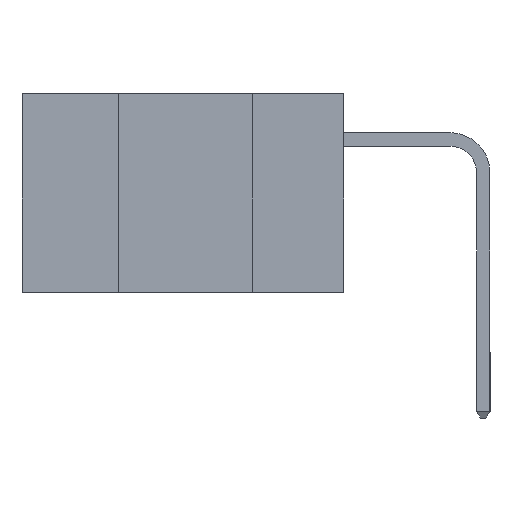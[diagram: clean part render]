
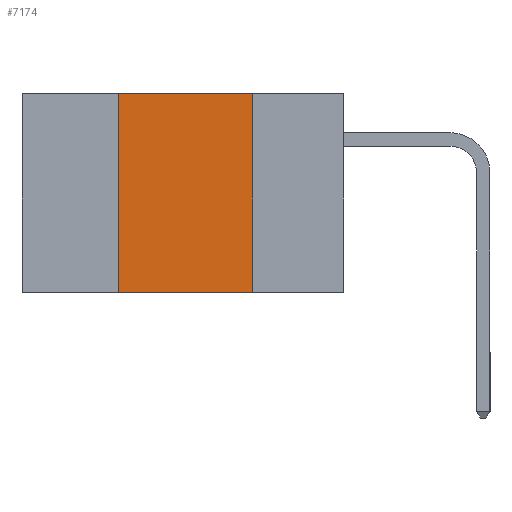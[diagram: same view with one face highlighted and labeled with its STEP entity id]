
A CAD part, left-side view. The second image highlights one B-rep face of the part: STEP entity #7174.
In plain terms, the highlighted planar face has unit normal (-1, 0, 0).
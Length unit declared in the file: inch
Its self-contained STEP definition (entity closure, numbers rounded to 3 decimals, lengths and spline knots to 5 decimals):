
#271 = DIRECTION ( 'NONE',  ( 0., -1., 0. ) ) ;
#311 = VERTEX_POINT ( 'NONE', #6300 ) ;
#550 = AXIS2_PLACEMENT_3D ( 'NONE', #8020, #4889, #9214 ) ;
#1442 = VECTOR ( 'NONE', #2116, 39.37008 ) ;
#1546 = ORIENTED_EDGE ( 'NONE', *, *, #4693, .T. ) ;
#2116 = DIRECTION ( 'NONE',  ( 0., 0., -1. ) ) ;
#2227 = DIRECTION ( 'NONE',  ( 0., 0., 1. ) ) ;
#2365 = CARTESIAN_POINT ( 'NONE',  ( 0., 0.42, -0.37 ) ) ;
#2449 = LINE ( 'NONE', #5404, #10309 ) ;
#3277 = EDGE_CURVE ( 'NONE', #311, #11477, #10362, .T. ) ;
#4693 = EDGE_CURVE ( 'NONE', #11360, #8022, #2449, .T. ) ;
#4889 = DIRECTION ( 'NONE',  ( 1., 0., 0. ) ) ;
#5208 = DIRECTION ( 'NONE',  ( 0., -1., 0. ) ) ;
#5230 = CARTESIAN_POINT ( 'NONE',  ( 0., 0.17, -0.37 ) ) ;
#5346 = EDGE_LOOP ( 'NONE', ( #12552, #11340, #6951, #1546 ) ) ;
#5404 = CARTESIAN_POINT ( 'NONE',  ( 0., 0.6, -0.37 ) ) ;
#5969 = PLANE ( 'NONE',  #550 ) ;
#6300 = CARTESIAN_POINT ( 'NONE',  ( 0., 0.42, 0. ) ) ;
#6310 = CARTESIAN_POINT ( 'NONE',  ( 0., 0.42, -0.37 ) ) ;
#6951 = ORIENTED_EDGE ( 'NONE', *, *, #7745, .F. ) ;
#7174 = ADVANCED_FACE ( 'NONE', ( #12876 ), #5969, .F. ) ;
#7241 = VECTOR ( 'NONE', #2227, 39.37008 ) ;
#7745 = EDGE_CURVE ( 'NONE', #11360, #311, #11630, .T. ) ;
#8020 = CARTESIAN_POINT ( 'NONE',  ( 0., 0.6, 0. ) ) ;
#8022 = VERTEX_POINT ( 'NONE', #5230 ) ;
#8134 = LINE ( 'NONE', #10101, #1442 ) ;
#8753 = EDGE_CURVE ( 'NONE', #11477, #8022, #8134, .T. ) ;
#9072 = VECTOR ( 'NONE', #5208, 39.37008 ) ;
#9214 = DIRECTION ( 'NONE',  ( 0., 0., -1. ) ) ;
#9627 = CARTESIAN_POINT ( 'NONE',  ( 0., 0.17, 0. ) ) ;
#10101 = CARTESIAN_POINT ( 'NONE',  ( 0., 0.17, -0.37 ) ) ;
#10309 = VECTOR ( 'NONE', #271, 39.37008 ) ;
#10362 = LINE ( 'NONE', #10427, #9072 ) ;
#10427 = CARTESIAN_POINT ( 'NONE',  ( 0., 0.6, 0. ) ) ;
#11340 = ORIENTED_EDGE ( 'NONE', *, *, #3277, .F. ) ;
#11360 = VERTEX_POINT ( 'NONE', #6310 ) ;
#11477 = VERTEX_POINT ( 'NONE', #9627 ) ;
#11630 = LINE ( 'NONE', #2365, #7241 ) ;
#12552 = ORIENTED_EDGE ( 'NONE', *, *, #8753, .F. ) ;
#12876 = FACE_OUTER_BOUND ( 'NONE', #5346, .T. ) ;
